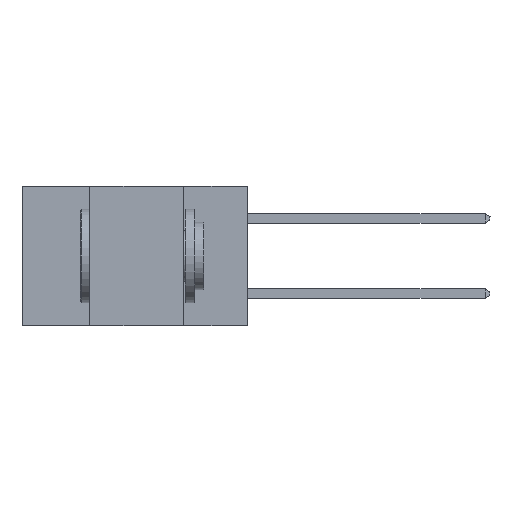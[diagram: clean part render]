
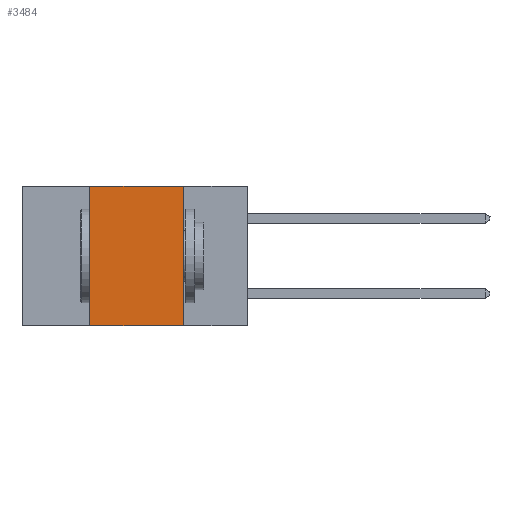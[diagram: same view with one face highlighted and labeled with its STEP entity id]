
A CAD part, left-side view. The second image highlights one B-rep face of the part: STEP entity #3484.
In plain terms, the highlighted planar face has unit normal (-1, 0, 0).
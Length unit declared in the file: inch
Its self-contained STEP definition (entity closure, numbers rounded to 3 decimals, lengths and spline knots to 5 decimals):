
#341 = ORIENTED_EDGE ( 'NONE', *, *, #3586, .T. ) ;
#795 = LINE ( 'NONE', #3944, #9151 ) ;
#1160 = LINE ( 'NONE', #1288, #3032 ) ;
#1288 = CARTESIAN_POINT ( 'NONE',  ( 0., 0.6, 0. ) ) ;
#1299 = DIRECTION ( 'NONE',  ( 1., 0., 0. ) ) ;
#2218 = ORIENTED_EDGE ( 'NONE', *, *, #3696, .F. ) ;
#3032 = VECTOR ( 'NONE', #10000, 39.37008 ) ;
#3122 = CARTESIAN_POINT ( 'NONE',  ( 0., 0.17, 0. ) ) ;
#3219 = VERTEX_POINT ( 'NONE', #4079 ) ;
#3484 = ADVANCED_FACE ( 'NONE', ( #4874 ), #8257, .F. ) ;
#3586 = EDGE_CURVE ( 'NONE', #3219, #9922, #795, .T. ) ;
#3696 = EDGE_CURVE ( 'NONE', #3219, #8569, #7438, .T. ) ;
#3769 = CARTESIAN_POINT ( 'NONE',  ( 0., 0.42, 0. ) ) ;
#3778 = ORIENTED_EDGE ( 'NONE', *, *, #7482, .F. ) ;
#3944 = CARTESIAN_POINT ( 'NONE',  ( 0., 0.6, -0.37 ) ) ;
#4079 = CARTESIAN_POINT ( 'NONE',  ( 0., 0.42, -0.37 ) ) ;
#4595 = DIRECTION ( 'NONE',  ( 0., 0., 1. ) ) ;
#4636 = CARTESIAN_POINT ( 'NONE',  ( 0., 0.42, 0. ) ) ;
#4874 = FACE_OUTER_BOUND ( 'NONE', #8679, .T. ) ;
#5028 = ORIENTED_EDGE ( 'NONE', *, *, #9177, .F. ) ;
#5047 = VECTOR ( 'NONE', #7038, 39.37008 ) ;
#6042 = CARTESIAN_POINT ( 'NONE',  ( 0., 0.6, 0. ) ) ;
#6080 = AXIS2_PLACEMENT_3D ( 'NONE', #6042, #1299, #6737 ) ;
#6138 = VERTEX_POINT ( 'NONE', #8921 ) ;
#6249 = CARTESIAN_POINT ( 'NONE',  ( 0., 0.17, -0.37 ) ) ;
#6737 = DIRECTION ( 'NONE',  ( 0., 0., -1. ) ) ;
#7038 = DIRECTION ( 'NONE',  ( 0., 0., -1. ) ) ;
#7438 = LINE ( 'NONE', #4636, #8887 ) ;
#7482 = EDGE_CURVE ( 'NONE', #6138, #9922, #9316, .T. ) ;
#8074 = DIRECTION ( 'NONE',  ( 0., -1., 0. ) ) ;
#8257 = PLANE ( 'NONE',  #6080 ) ;
#8569 = VERTEX_POINT ( 'NONE', #3769 ) ;
#8679 = EDGE_LOOP ( 'NONE', ( #3778, #5028, #2218, #341 ) ) ;
#8887 = VECTOR ( 'NONE', #4595, 39.37008 ) ;
#8921 = CARTESIAN_POINT ( 'NONE',  ( 0., 0.17, 0. ) ) ;
#9151 = VECTOR ( 'NONE', #8074, 39.37008 ) ;
#9177 = EDGE_CURVE ( 'NONE', #8569, #6138, #1160, .T. ) ;
#9316 = LINE ( 'NONE', #3122, #5047 ) ;
#9922 = VERTEX_POINT ( 'NONE', #6249 ) ;
#10000 = DIRECTION ( 'NONE',  ( 0., -1., 0. ) ) ;
